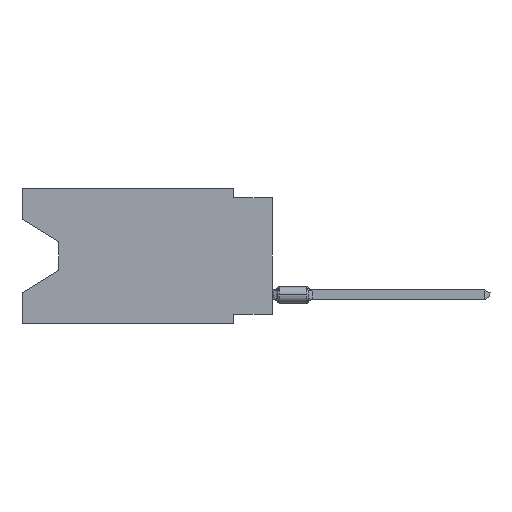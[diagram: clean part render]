
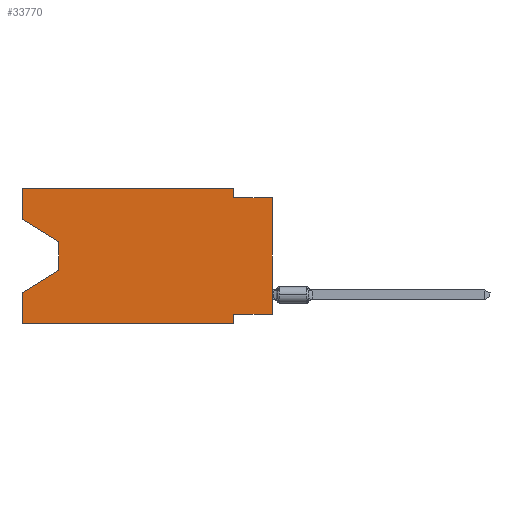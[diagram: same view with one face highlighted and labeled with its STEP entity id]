
A CAD part, left-side view. The second image highlights one B-rep face of the part: STEP entity #33770.
In plain terms, the highlighted planar face has unit normal (-1, 0, 0).
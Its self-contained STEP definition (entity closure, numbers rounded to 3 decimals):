
#463 = CARTESIAN_POINT ( 'NONE',  ( 0., 13.97, -3.505 ) ) ;
#862 = CARTESIAN_POINT ( 'NONE',  ( 0., 2.54, -8.89 ) ) ;
#1357 = DIRECTION ( 'NONE',  ( 0., -0.855, -0.519 ) ) ;
#2031 = LINE ( 'NONE', #19401, #24872 ) ;
#2065 = VECTOR ( 'NONE', #44742, 1000. ) ;
#2181 = VECTOR ( 'NONE', #28250, 1000. ) ;
#2245 = VERTEX_POINT ( 'NONE', #28957 ) ;
#3370 = CARTESIAN_POINT ( 'NONE',  ( 0., 0., -0.635 ) ) ;
#3923 = EDGE_CURVE ( 'NONE', #28743, #23917, #29642, .T. ) ;
#4192 = ORIENTED_EDGE ( 'NONE', *, *, #9786, .F. ) ;
#4252 = CARTESIAN_POINT ( 'NONE',  ( 0., 2.54, 0. ) ) ;
#4668 = VECTOR ( 'NONE', #15663, 1000. ) ;
#5206 = EDGE_CURVE ( 'NONE', #13620, #31828, #37846, .T. ) ;
#5355 = CARTESIAN_POINT ( 'NONE',  ( 0., 0., -8.255 ) ) ;
#5359 = VECTOR ( 'NONE', #8495, 1000. ) ;
#5901 = CARTESIAN_POINT ( 'NONE',  ( 0., 2.54, 0. ) ) ;
#6350 = DIRECTION ( 'NONE',  ( 0., 0.855, -0.519 ) ) ;
#7855 = CARTESIAN_POINT ( 'NONE',  ( 0., 16.383, -8.89 ) ) ;
#8106 = EDGE_CURVE ( 'NONE', #31828, #11317, #33331, .T. ) ;
#8495 = DIRECTION ( 'NONE',  ( 0., -1., 0. ) ) ;
#9047 = LINE ( 'NONE', #12233, #20948 ) ;
#9399 = VERTEX_POINT ( 'NONE', #862 ) ;
#9786 = EDGE_CURVE ( 'NONE', #14949, #13620, #21364, .T. ) ;
#10000 = VERTEX_POINT ( 'NONE', #33848 ) ;
#10269 = ORIENTED_EDGE ( 'NONE', *, *, #13246, .T. ) ;
#10430 = CARTESIAN_POINT ( 'NONE',  ( 0., 2.54, -0.635 ) ) ;
#11317 = VERTEX_POINT ( 'NONE', #3370 ) ;
#12233 = CARTESIAN_POINT ( 'NONE',  ( 0., 0., -8.255 ) ) ;
#12281 = DIRECTION ( 'NONE',  ( 0., 0., -1. ) ) ;
#12782 = CARTESIAN_POINT ( 'NONE',  ( 0., 16.383, -2.038 ) ) ;
#12849 = LINE ( 'NONE', #13076, #42787 ) ;
#13076 = CARTESIAN_POINT ( 'NONE',  ( 0., 16.383, 0. ) ) ;
#13246 = EDGE_CURVE ( 'NONE', #23917, #10000, #16633, .T. ) ;
#13620 = VERTEX_POINT ( 'NONE', #4252 ) ;
#13701 = EDGE_CURVE ( 'NONE', #22198, #2245, #9047, .T. ) ;
#14128 = CARTESIAN_POINT ( 'NONE',  ( 0., 0., -0.635 ) ) ;
#14317 = LINE ( 'NONE', #25283, #2181 ) ;
#14949 = VERTEX_POINT ( 'NONE', #43990 ) ;
#15663 = DIRECTION ( 'NONE',  ( 0., 0., -1. ) ) ;
#16468 = EDGE_CURVE ( 'NONE', #22198, #11317, #30550, .T. ) ;
#16633 = LINE ( 'NONE', #19616, #18746 ) ;
#17653 = DIRECTION ( 'NONE',  ( 0., 0., -1. ) ) ;
#17868 = VERTEX_POINT ( 'NONE', #7855 ) ;
#18735 = LINE ( 'NONE', #32637, #40578 ) ;
#18746 = VECTOR ( 'NONE', #6350, 1000. ) ;
#18887 = EDGE_LOOP ( 'NONE', ( #42682, #22393, #10269, #23513, #33955, #20135, #19611, #28854, #37231, #22228, #4192, #35960 ) ) ;
#18959 = DIRECTION ( 'NONE',  ( 0., -1., 0. ) ) ;
#18976 = EDGE_CURVE ( 'NONE', #39075, #14949, #12849, .T. ) ;
#19401 = CARTESIAN_POINT ( 'NONE',  ( 0., 16.383, -8.89 ) ) ;
#19611 = ORIENTED_EDGE ( 'NONE', *, *, #13701, .F. ) ;
#19616 = CARTESIAN_POINT ( 'NONE',  ( 0., 13.97, -5.385 ) ) ;
#20135 = ORIENTED_EDGE ( 'NONE', *, *, #25122, .F. ) ;
#20521 = CARTESIAN_POINT ( 'NONE',  ( 0., 0., 0. ) ) ;
#20740 = DIRECTION ( 'NONE',  ( 0., 0., -1. ) ) ;
#20948 = VECTOR ( 'NONE', #22753, 1000. ) ;
#21061 = FACE_OUTER_BOUND ( 'NONE', #18887, .T. ) ;
#21364 = LINE ( 'NONE', #25024, #5359 ) ;
#21997 = CARTESIAN_POINT ( 'NONE',  ( 0., 13.97, -5.385 ) ) ;
#22198 = VERTEX_POINT ( 'NONE', #5355 ) ;
#22228 = ORIENTED_EDGE ( 'NONE', *, *, #5206, .F. ) ;
#22393 = ORIENTED_EDGE ( 'NONE', *, *, #3923, .T. ) ;
#22753 = DIRECTION ( 'NONE',  ( 0., 1., 0. ) ) ;
#23157 = VECTOR ( 'NONE', #20740, 1000. ) ;
#23372 = EDGE_CURVE ( 'NONE', #39075, #28743, #18735, .T. ) ;
#23513 = ORIENTED_EDGE ( 'NONE', *, *, #34718, .F. ) ;
#23917 = VERTEX_POINT ( 'NONE', #21997 ) ;
#24046 = CARTESIAN_POINT ( 'NONE',  ( 0., 16.383, 0. ) ) ;
#24872 = VECTOR ( 'NONE', #18959, 1000. ) ;
#25024 = CARTESIAN_POINT ( 'NONE',  ( 0., 16.383, 0. ) ) ;
#25122 = EDGE_CURVE ( 'NONE', #2245, #9399, #33013, .T. ) ;
#25283 = CARTESIAN_POINT ( 'NONE',  ( 0., 16.383, 0. ) ) ;
#26153 = CARTESIAN_POINT ( 'NONE',  ( 0., 2.54, -8.89 ) ) ;
#28250 = DIRECTION ( 'NONE',  ( 0., 0., 1. ) ) ;
#28743 = VERTEX_POINT ( 'NONE', #463 ) ;
#28854 = ORIENTED_EDGE ( 'NONE', *, *, #16468, .T. ) ;
#28957 = CARTESIAN_POINT ( 'NONE',  ( 0., 2.54, -8.255 ) ) ;
#29642 = LINE ( 'NONE', #43562, #43587 ) ;
#30331 = DIRECTION ( 'NONE',  ( 0., 0., 1. ) ) ;
#30550 = LINE ( 'NONE', #20521, #43650 ) ;
#31828 = VERTEX_POINT ( 'NONE', #10430 ) ;
#32637 = CARTESIAN_POINT ( 'NONE',  ( 0., 16.383, -2.038 ) ) ;
#33013 = LINE ( 'NONE', #26153, #4668 ) ;
#33331 = LINE ( 'NONE', #14128, #2065 ) ;
#33770 = ADVANCED_FACE ( 'NONE', ( #21061 ), #34326, .F. ) ;
#33848 = CARTESIAN_POINT ( 'NONE',  ( 0., 16.383, -6.852 ) ) ;
#33955 = ORIENTED_EDGE ( 'NONE', *, *, #35719, .T. ) ;
#34326 = PLANE ( 'NONE',  #39418 ) ;
#34718 = EDGE_CURVE ( 'NONE', #17868, #10000, #14317, .T. ) ;
#35719 = EDGE_CURVE ( 'NONE', #17868, #9399, #2031, .T. ) ;
#35960 = ORIENTED_EDGE ( 'NONE', *, *, #18976, .F. ) ;
#37231 = ORIENTED_EDGE ( 'NONE', *, *, #8106, .F. ) ;
#37846 = LINE ( 'NONE', #5901, #23157 ) ;
#37979 = DIRECTION ( 'NONE',  ( 1., 0., 0. ) ) ;
#39075 = VERTEX_POINT ( 'NONE', #12782 ) ;
#39418 = AXIS2_PLACEMENT_3D ( 'NONE', #24046, #37979, #17653 ) ;
#40578 = VECTOR ( 'NONE', #1357, 1000. ) ;
#41172 = DIRECTION ( 'NONE',  ( 0., 0., 1. ) ) ;
#42682 = ORIENTED_EDGE ( 'NONE', *, *, #23372, .T. ) ;
#42787 = VECTOR ( 'NONE', #41172, 1000. ) ;
#43562 = CARTESIAN_POINT ( 'NONE',  ( 0., 13.97, -3.505 ) ) ;
#43587 = VECTOR ( 'NONE', #12281, 1000. ) ;
#43650 = VECTOR ( 'NONE', #30331, 1000. ) ;
#43990 = CARTESIAN_POINT ( 'NONE',  ( 0., 16.383, 0. ) ) ;
#44742 = DIRECTION ( 'NONE',  ( 0., -1., 0. ) ) ;
